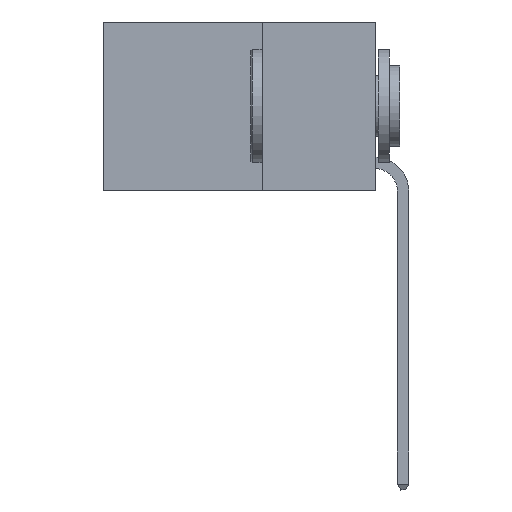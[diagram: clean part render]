
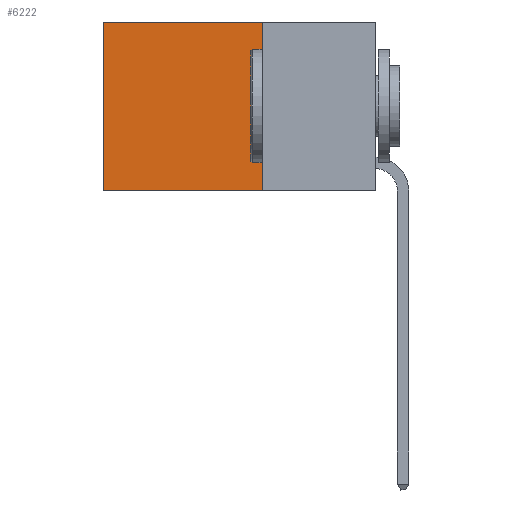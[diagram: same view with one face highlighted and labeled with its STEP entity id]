
A CAD part, left-side view. The second image highlights one B-rep face of the part: STEP entity #6222.
In plain terms, the highlighted planar face has unit normal (-1, 0, 0).
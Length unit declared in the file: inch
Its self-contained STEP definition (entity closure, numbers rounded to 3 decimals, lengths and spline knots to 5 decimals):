
#210 = FACE_OUTER_BOUND ( 'NONE', #1895, .T. ) ;
#680 = LINE ( 'NONE', #5619, #14550 ) ;
#1428 = DIRECTION ( 'NONE',  ( 0., 1., 0. ) ) ;
#1786 = VECTOR ( 'NONE', #4828, 39.37008 ) ;
#1895 = EDGE_LOOP ( 'NONE', ( #9475, #14810, #12573, #3454 ) ) ;
#2759 = LINE ( 'NONE', #4038, #6323 ) ;
#2927 = EDGE_CURVE ( 'NONE', #13737, #10259, #7322, .T. ) ;
#3332 = VERTEX_POINT ( 'NONE', #5973 ) ;
#3454 = ORIENTED_EDGE ( 'NONE', *, *, #3633, .T. ) ;
#3633 = EDGE_CURVE ( 'NONE', #13737, #4077, #680, .T. ) ;
#4038 = CARTESIAN_POINT ( 'NONE',  ( 0.2625, 0.25, -0.37 ) ) ;
#4077 = VERTEX_POINT ( 'NONE', #15396 ) ;
#4828 = DIRECTION ( 'NONE',  ( 0., 0., -1. ) ) ;
#4916 = DIRECTION ( 'NONE',  ( 0., 0., -1. ) ) ;
#5083 = DIRECTION ( 'NONE',  ( 1., 0., 0. ) ) ;
#5619 = CARTESIAN_POINT ( 'NONE',  ( 0.2625, 0.25, 0. ) ) ;
#5973 = CARTESIAN_POINT ( 'NONE',  ( 0.2625, 0.6, -0.37 ) ) ;
#6073 = CARTESIAN_POINT ( 'NONE',  ( 0.2625, 0.25, 0. ) ) ;
#6222 = ADVANCED_FACE ( 'NONE', ( #210 ), #6407, .F. ) ;
#6323 = VECTOR ( 'NONE', #1428, 39.37008 ) ;
#6407 = PLANE ( 'NONE',  #14861 ) ;
#6535 = EDGE_CURVE ( 'NONE', #10259, #3332, #2759, .T. ) ;
#7322 = LINE ( 'NONE', #6073, #14336 ) ;
#7575 = LINE ( 'NONE', #16444, #1786 ) ;
#8653 = EDGE_CURVE ( 'NONE', #4077, #3332, #7575, .T. ) ;
#9081 = DIRECTION ( 'NONE',  ( 0., 0., -1. ) ) ;
#9475 = ORIENTED_EDGE ( 'NONE', *, *, #8653, .T. ) ;
#10259 = VERTEX_POINT ( 'NONE', #15921 ) ;
#12573 = ORIENTED_EDGE ( 'NONE', *, *, #2927, .F. ) ;
#13024 = CARTESIAN_POINT ( 'NONE',  ( 0.2625, 0.25, 0. ) ) ;
#13737 = VERTEX_POINT ( 'NONE', #13024 ) ;
#14336 = VECTOR ( 'NONE', #4916, 39.37008 ) ;
#14550 = VECTOR ( 'NONE', #15986, 39.37008 ) ;
#14810 = ORIENTED_EDGE ( 'NONE', *, *, #6535, .F. ) ;
#14861 = AXIS2_PLACEMENT_3D ( 'NONE', #16535, #5083, #9081 ) ;
#15396 = CARTESIAN_POINT ( 'NONE',  ( 0.2625, 0.6, 0. ) ) ;
#15921 = CARTESIAN_POINT ( 'NONE',  ( 0.2625, 0.25, -0.37 ) ) ;
#15986 = DIRECTION ( 'NONE',  ( 0., 1., 0. ) ) ;
#16444 = CARTESIAN_POINT ( 'NONE',  ( 0.2625, 0.6, 0. ) ) ;
#16535 = CARTESIAN_POINT ( 'NONE',  ( 0.2625, 0.25, 0. ) ) ;
